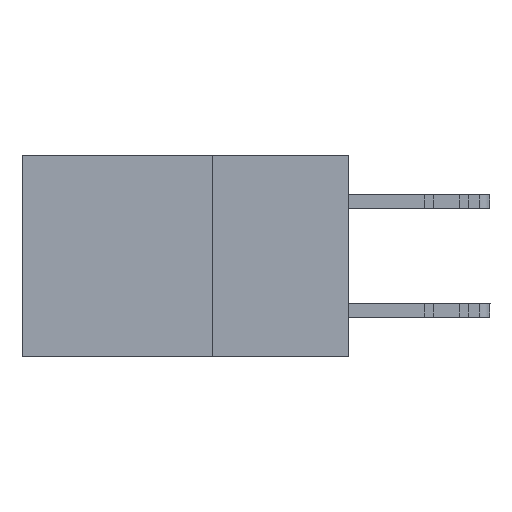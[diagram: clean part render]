
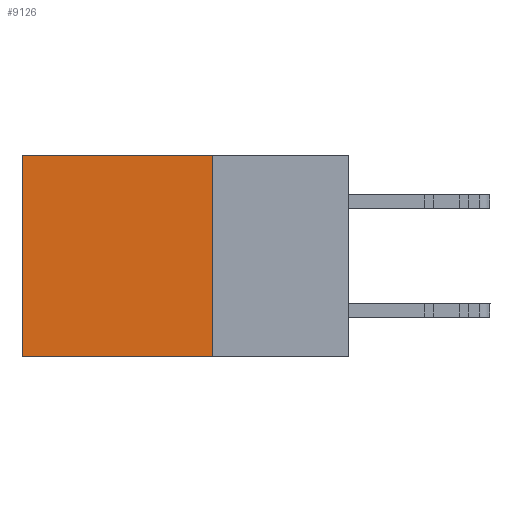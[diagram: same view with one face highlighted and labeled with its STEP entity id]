
A CAD part, left-side view. The second image highlights one B-rep face of the part: STEP entity #9126.
In plain terms, the highlighted planar face has unit normal (-1, 0, 0).
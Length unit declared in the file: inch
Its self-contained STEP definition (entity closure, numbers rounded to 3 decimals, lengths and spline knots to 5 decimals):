
#220 = CARTESIAN_POINT ( 'NONE',  ( 0.298, 0.25, -0.37 ) ) ;
#2173 = EDGE_LOOP ( 'NONE', ( #22142, #26059, #11226, #5321 ) ) ;
#2443 = CARTESIAN_POINT ( 'NONE',  ( 0.298, 0.25, 0. ) ) ;
#2812 = VERTEX_POINT ( 'NONE', #28432 ) ;
#3523 = VERTEX_POINT ( 'NONE', #220 ) ;
#5321 = ORIENTED_EDGE ( 'NONE', *, *, #15459, .T. ) ;
#7236 = VECTOR ( 'NONE', #28447, 39.37008 ) ;
#8109 = FACE_OUTER_BOUND ( 'NONE', #2173, .T. ) ;
#9126 = ADVANCED_FACE ( 'NONE', ( #8109 ), #12380, .F. ) ;
#9127 = CARTESIAN_POINT ( 'NONE',  ( 0.298, 0.25, -0.37 ) ) ;
#9177 = VECTOR ( 'NONE', #26174, 39.37008 ) ;
#9669 = EDGE_CURVE ( 'NONE', #13686, #3523, #18024, .T. ) ;
#11226 = ORIENTED_EDGE ( 'NONE', *, *, #9669, .F. ) ;
#11920 = EDGE_CURVE ( 'NONE', #3523, #12317, #22487, .T. ) ;
#12317 = VERTEX_POINT ( 'NONE', #23108 ) ;
#12380 = PLANE ( 'NONE',  #27450 ) ;
#13092 = DIRECTION ( 'NONE',  ( 0., 1., 0. ) ) ;
#13686 = VERTEX_POINT ( 'NONE', #14326 ) ;
#14030 = VECTOR ( 'NONE', #25643, 39.37008 ) ;
#14326 = CARTESIAN_POINT ( 'NONE',  ( 0.298, 0.25, 0. ) ) ;
#14604 = LINE ( 'NONE', #21188, #7236 ) ;
#15047 = DIRECTION ( 'NONE',  ( 1., 0., 0. ) ) ;
#15459 = EDGE_CURVE ( 'NONE', #13686, #2812, #25290, .T. ) ;
#16031 = VECTOR ( 'NONE', #13092, 39.37008 ) ;
#18024 = LINE ( 'NONE', #2443, #9177 ) ;
#19680 = DIRECTION ( 'NONE',  ( 0., 0., -1. ) ) ;
#21188 = CARTESIAN_POINT ( 'NONE',  ( 0.298, 0.6, 0. ) ) ;
#22142 = ORIENTED_EDGE ( 'NONE', *, *, #30007, .T. ) ;
#22440 = CARTESIAN_POINT ( 'NONE',  ( 0.298, 0.25, 0. ) ) ;
#22487 = LINE ( 'NONE', #9127, #14030 ) ;
#23108 = CARTESIAN_POINT ( 'NONE',  ( 0.298, 0.6, -0.37 ) ) ;
#25290 = LINE ( 'NONE', #22440, #16031 ) ;
#25643 = DIRECTION ( 'NONE',  ( 0., 1., 0. ) ) ;
#26059 = ORIENTED_EDGE ( 'NONE', *, *, #11920, .F. ) ;
#26174 = DIRECTION ( 'NONE',  ( 0., 0., -1. ) ) ;
#26601 = CARTESIAN_POINT ( 'NONE',  ( 0.298, 0.25, 0. ) ) ;
#27450 = AXIS2_PLACEMENT_3D ( 'NONE', #26601, #15047, #19680 ) ;
#28432 = CARTESIAN_POINT ( 'NONE',  ( 0.298, 0.6, 0. ) ) ;
#28447 = DIRECTION ( 'NONE',  ( 0., 0., -1. ) ) ;
#30007 = EDGE_CURVE ( 'NONE', #2812, #12317, #14604, .T. ) ;
